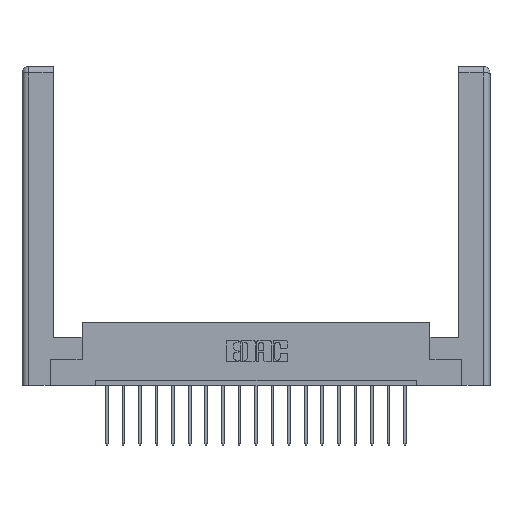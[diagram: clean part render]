
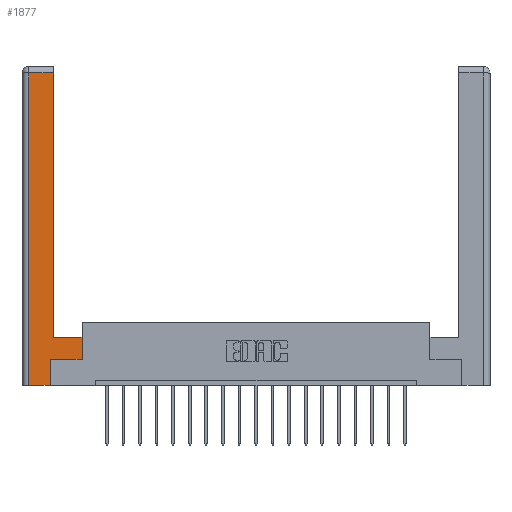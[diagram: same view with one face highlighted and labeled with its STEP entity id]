
A CAD part, top view. The second image highlights one B-rep face of the part: STEP entity #1877.
In plain terms, the highlighted planar face has unit normal (0, 0, 1).
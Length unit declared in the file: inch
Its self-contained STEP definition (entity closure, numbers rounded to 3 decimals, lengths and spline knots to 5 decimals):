
#144 = CARTESIAN_POINT ( 'NONE',  ( 0.0615, 0., 0. ) ) ;
#722 = VERTEX_POINT ( 'NONE', #144 ) ;
#742 = CARTESIAN_POINT ( 'NONE',  ( 0.265, 0.245, 0. ) ) ;
#872 = EDGE_CURVE ( 'NONE', #17436, #19189, #3608, .T. ) ;
#1496 = VERTEX_POINT ( 'NONE', #19134 ) ;
#1680 = VECTOR ( 'NONE', #12825, 39.37008 ) ;
#1687 = DIRECTION ( 'NONE',  ( -1., 0., 0. ) ) ;
#1877 = ADVANCED_FACE ( 'NONE', ( #15267 ), #15395, .F. ) ;
#1962 = VECTOR ( 'NONE', #11483, 39.37008 ) ;
#2464 = DIRECTION ( 'NONE',  ( 1., 0., 0. ) ) ;
#2706 = EDGE_LOOP ( 'NONE', ( #18124, #15422, #5314, #10222, #6806, #3321, #11431, #12196 ) ) ;
#2777 = EDGE_CURVE ( 'NONE', #16604, #17367, #6135, .T. ) ;
#3063 = CARTESIAN_POINT ( 'NONE',  ( 0.565, 0.45, 0. ) ) ;
#3157 = VERTEX_POINT ( 'NONE', #14997 ) ;
#3321 = ORIENTED_EDGE ( 'NONE', *, *, #5652, .T. ) ;
#3608 = LINE ( 'NONE', #742, #1680 ) ;
#3926 = VECTOR ( 'NONE', #18013, 39.37008 ) ;
#4344 = AXIS2_PLACEMENT_3D ( 'NONE', #4763, #10831, #1687 ) ;
#4763 = CARTESIAN_POINT ( 'NONE',  ( 0., 0., 0. ) ) ;
#5314 = ORIENTED_EDGE ( 'NONE', *, *, #9765, .T. ) ;
#5533 = CARTESIAN_POINT ( 'NONE',  ( 0.265, 0., 0. ) ) ;
#5652 = EDGE_CURVE ( 'NONE', #19189, #3157, #8452, .T. ) ;
#5959 = CARTESIAN_POINT ( 'NONE',  ( 0.565, 0.245, 0. ) ) ;
#6001 = DIRECTION ( 'NONE',  ( 0., -1., 0. ) ) ;
#6135 = LINE ( 'NONE', #17207, #14274 ) ;
#6806 = ORIENTED_EDGE ( 'NONE', *, *, #872, .T. ) ;
#7280 = CARTESIAN_POINT ( 'NONE',  ( 0.295, 2.94, 0. ) ) ;
#7446 = LINE ( 'NONE', #13239, #1962 ) ;
#7523 = VECTOR ( 'NONE', #19754, 39.37008 ) ;
#7726 = VECTOR ( 'NONE', #6001, 39.37008 ) ;
#8215 = VECTOR ( 'NONE', #2464, 39.37008 ) ;
#8452 = LINE ( 'NONE', #5959, #3926 ) ;
#8550 = LINE ( 'NONE', #3063, #10198 ) ;
#8697 = LINE ( 'NONE', #16367, #8215 ) ;
#9765 = EDGE_CURVE ( 'NONE', #1496, #722, #17044, .T. ) ;
#10198 = VECTOR ( 'NONE', #18175, 39.37008 ) ;
#10207 = EDGE_CURVE ( 'NONE', #13824, #16604, #7446, .T. ) ;
#10222 = ORIENTED_EDGE ( 'NONE', *, *, #16052, .T. ) ;
#10831 = DIRECTION ( 'NONE',  ( 0., 0., -1. ) ) ;
#11431 = ORIENTED_EDGE ( 'NONE', *, *, #13762, .T. ) ;
#11483 = DIRECTION ( 'NONE',  ( -1., 0., 0. ) ) ;
#12052 = LINE ( 'NONE', #13753, #7523 ) ;
#12159 = CARTESIAN_POINT ( 'NONE',  ( 0.295, 0.45, 0. ) ) ;
#12196 = ORIENTED_EDGE ( 'NONE', *, *, #10207, .T. ) ;
#12825 = DIRECTION ( 'NONE',  ( 0., 1., 0. ) ) ;
#13239 = CARTESIAN_POINT ( 'NONE',  ( 0.295, 0.45, 0. ) ) ;
#13753 = CARTESIAN_POINT ( 'NONE',  ( 0.0615, 2.94, 0. ) ) ;
#13762 = EDGE_CURVE ( 'NONE', #3157, #13824, #8550, .T. ) ;
#13824 = VERTEX_POINT ( 'NONE', #17368 ) ;
#14274 = VECTOR ( 'NONE', #15629, 39.37008 ) ;
#14997 = CARTESIAN_POINT ( 'NONE',  ( 0.565, 0.245, 0. ) ) ;
#15267 = FACE_OUTER_BOUND ( 'NONE', #2706, .T. ) ;
#15395 = PLANE ( 'NONE',  #4344 ) ;
#15422 = ORIENTED_EDGE ( 'NONE', *, *, #19257, .T. ) ;
#15629 = DIRECTION ( 'NONE',  ( 0., 1., 0. ) ) ;
#16052 = EDGE_CURVE ( 'NONE', #722, #17436, #8697, .T. ) ;
#16367 = CARTESIAN_POINT ( 'NONE',  ( 0.265, 0., 0. ) ) ;
#16604 = VERTEX_POINT ( 'NONE', #12159 ) ;
#16642 = CARTESIAN_POINT ( 'NONE',  ( 0.0615, 0., 0. ) ) ;
#17044 = LINE ( 'NONE', #16642, #7726 ) ;
#17207 = CARTESIAN_POINT ( 'NONE',  ( 0.295, 3., 0. ) ) ;
#17367 = VERTEX_POINT ( 'NONE', #7280 ) ;
#17368 = CARTESIAN_POINT ( 'NONE',  ( 0.565, 0.45, 0. ) ) ;
#17436 = VERTEX_POINT ( 'NONE', #5533 ) ;
#18013 = DIRECTION ( 'NONE',  ( 1., 0., 0. ) ) ;
#18124 = ORIENTED_EDGE ( 'NONE', *, *, #2777, .T. ) ;
#18175 = DIRECTION ( 'NONE',  ( 0., 1., 0. ) ) ;
#19134 = CARTESIAN_POINT ( 'NONE',  ( 0.0615, 2.94, 0. ) ) ;
#19189 = VERTEX_POINT ( 'NONE', #19429 ) ;
#19257 = EDGE_CURVE ( 'NONE', #17367, #1496, #12052, .T. ) ;
#19429 = CARTESIAN_POINT ( 'NONE',  ( 0.265, 0.245, 0. ) ) ;
#19754 = DIRECTION ( 'NONE',  ( -1., 0., 0. ) ) ;
